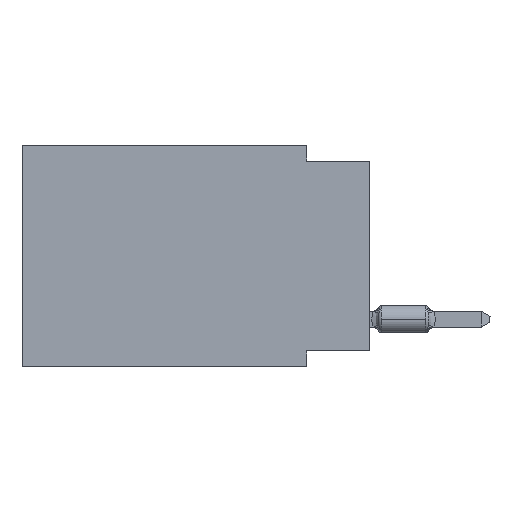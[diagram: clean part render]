
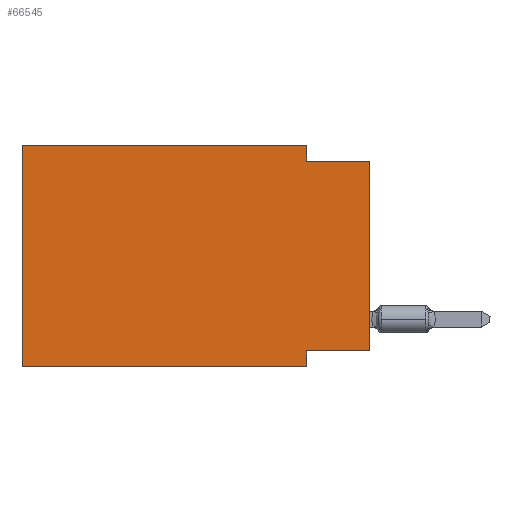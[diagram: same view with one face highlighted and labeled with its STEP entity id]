
A CAD part, left-side view. The second image highlights one B-rep face of the part: STEP entity #66545.
In plain terms, the highlighted planar face has unit normal (-1, 0, 0).
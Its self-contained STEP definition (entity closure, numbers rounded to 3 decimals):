
#882 = EDGE_CURVE ( 'NONE', #19711, #16818, #31482, .T. ) ;
#2258 = CARTESIAN_POINT ( 'NONE',  ( 0., 0., -8.255 ) ) ;
#3545 = DIRECTION ( 'NONE',  ( 0., 0., -1. ) ) ;
#5819 = EDGE_CURVE ( 'NONE', #34716, #10950, #70149, .T. ) ;
#7130 = VECTOR ( 'NONE', #69874, 1000. ) ;
#8176 = EDGE_CURVE ( 'NONE', #34716, #53048, #27518, .T. ) ;
#9474 = PLANE ( 'NONE',  #44403 ) ;
#9476 = CARTESIAN_POINT ( 'NONE',  ( 0., 13.97, 0. ) ) ;
#9619 = VECTOR ( 'NONE', #11714, 1000. ) ;
#10744 = EDGE_CURVE ( 'NONE', #30402, #53048, #65642, .T. ) ;
#10950 = VERTEX_POINT ( 'NONE', #67237 ) ;
#11714 = DIRECTION ( 'NONE',  ( 0., -1., 0. ) ) ;
#12841 = VECTOR ( 'NONE', #71300, 1000. ) ;
#14207 = DIRECTION ( 'NONE',  ( 0., 0., 1. ) ) ;
#15146 = FACE_OUTER_BOUND ( 'NONE', #59565, .T. ) ;
#15240 = CARTESIAN_POINT ( 'NONE',  ( 0., 2.54, 0. ) ) ;
#16005 = VECTOR ( 'NONE', #77362, 1000. ) ;
#16038 = LINE ( 'NONE', #64950, #45144 ) ;
#16060 = CARTESIAN_POINT ( 'NONE',  ( 0., 0., -8.255 ) ) ;
#16818 = VERTEX_POINT ( 'NONE', #61718 ) ;
#18190 = LINE ( 'NONE', #31099, #9619 ) ;
#19505 = EDGE_CURVE ( 'NONE', #75774, #48635, #18190, .T. ) ;
#19711 = VERTEX_POINT ( 'NONE', #63715 ) ;
#25795 = CARTESIAN_POINT ( 'NONE',  ( 0., 0., -0.635 ) ) ;
#27288 = DIRECTION ( 'NONE',  ( 0., 1., 0. ) ) ;
#27518 = LINE ( 'NONE', #75637, #36383 ) ;
#30402 = VERTEX_POINT ( 'NONE', #72720 ) ;
#31099 = CARTESIAN_POINT ( 'NONE',  ( 0., 13.97, 0. ) ) ;
#31482 = LINE ( 'NONE', #32697, #7130 ) ;
#32697 = CARTESIAN_POINT ( 'NONE',  ( 0., 13.97, -8.89 ) ) ;
#33601 = ORIENTED_EDGE ( 'NONE', *, *, #35800, .F. ) ;
#34716 = VERTEX_POINT ( 'NONE', #16060 ) ;
#35800 = EDGE_CURVE ( 'NONE', #48635, #30402, #16038, .T. ) ;
#36383 = VECTOR ( 'NONE', #14207, 1000. ) ;
#38687 = ORIENTED_EDGE ( 'NONE', *, *, #8176, .T. ) ;
#43148 = CARTESIAN_POINT ( 'NONE',  ( 0., 2.54, -8.89 ) ) ;
#44403 = AXIS2_PLACEMENT_3D ( 'NONE', #57993, #53127, #70128 ) ;
#45144 = VECTOR ( 'NONE', #3545, 1000. ) ;
#46657 = LINE ( 'NONE', #9476, #12841 ) ;
#47250 = EDGE_CURVE ( 'NONE', #10950, #16818, #55284, .T. ) ;
#47547 = CARTESIAN_POINT ( 'NONE',  ( 0., 13.97, 0. ) ) ;
#48635 = VERTEX_POINT ( 'NONE', #15240 ) ;
#50139 = ORIENTED_EDGE ( 'NONE', *, *, #5819, .F. ) ;
#53048 = VERTEX_POINT ( 'NONE', #69501 ) ;
#53127 = DIRECTION ( 'NONE',  ( 1., 0., 0. ) ) ;
#54773 = ORIENTED_EDGE ( 'NONE', *, *, #47250, .F. ) ;
#55284 = LINE ( 'NONE', #43148, #65411 ) ;
#57993 = CARTESIAN_POINT ( 'NONE',  ( 0., 13.97, 0. ) ) ;
#58066 = ORIENTED_EDGE ( 'NONE', *, *, #882, .T. ) ;
#59565 = EDGE_LOOP ( 'NONE', ( #38687, #67323, #33601, #79434, #73044, #58066, #54773, #50139 ) ) ;
#61718 = CARTESIAN_POINT ( 'NONE',  ( 0., 2.54, -8.89 ) ) ;
#63715 = CARTESIAN_POINT ( 'NONE',  ( 0., 13.97, -8.89 ) ) ;
#64950 = CARTESIAN_POINT ( 'NONE',  ( 0., 2.54, 0. ) ) ;
#65411 = VECTOR ( 'NONE', #79921, 1000. ) ;
#65642 = LINE ( 'NONE', #25795, #16005 ) ;
#66545 = ADVANCED_FACE ( 'NONE', ( #15146 ), #9474, .F. ) ;
#67237 = CARTESIAN_POINT ( 'NONE',  ( 0., 2.54, -8.255 ) ) ;
#67323 = ORIENTED_EDGE ( 'NONE', *, *, #10744, .F. ) ;
#69501 = CARTESIAN_POINT ( 'NONE',  ( 0., 0., -0.635 ) ) ;
#69874 = DIRECTION ( 'NONE',  ( 0., -1., 0. ) ) ;
#70128 = DIRECTION ( 'NONE',  ( 0., 0., -1. ) ) ;
#70149 = LINE ( 'NONE', #2258, #78751 ) ;
#71300 = DIRECTION ( 'NONE',  ( 0., 0., 1. ) ) ;
#72720 = CARTESIAN_POINT ( 'NONE',  ( 0., 2.54, -0.635 ) ) ;
#73044 = ORIENTED_EDGE ( 'NONE', *, *, #77434, .F. ) ;
#75637 = CARTESIAN_POINT ( 'NONE',  ( 0., 0., 0. ) ) ;
#75774 = VERTEX_POINT ( 'NONE', #47547 ) ;
#77362 = DIRECTION ( 'NONE',  ( 0., -1., 0. ) ) ;
#77434 = EDGE_CURVE ( 'NONE', #19711, #75774, #46657, .T. ) ;
#78751 = VECTOR ( 'NONE', #27288, 1000. ) ;
#79434 = ORIENTED_EDGE ( 'NONE', *, *, #19505, .F. ) ;
#79921 = DIRECTION ( 'NONE',  ( 0., 0., -1. ) ) ;
